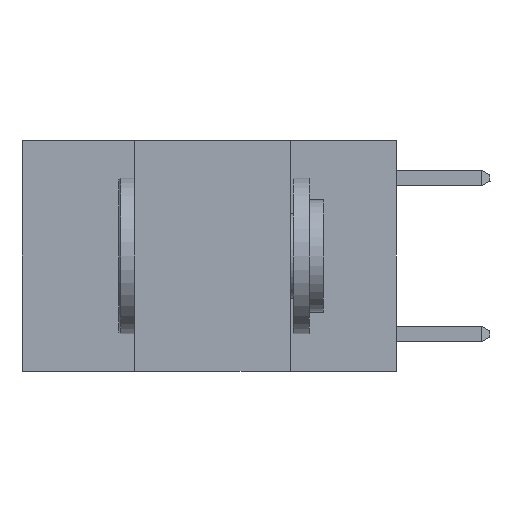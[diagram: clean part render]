
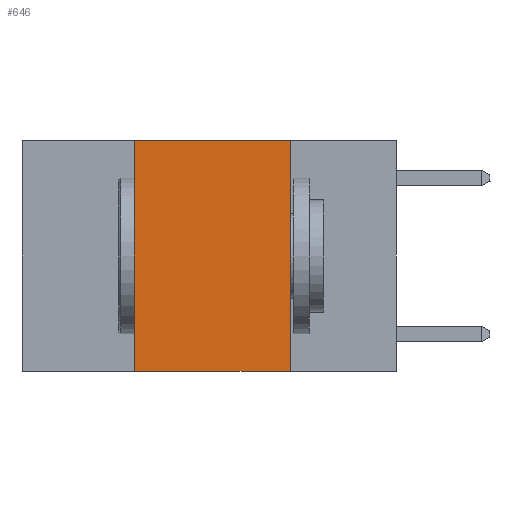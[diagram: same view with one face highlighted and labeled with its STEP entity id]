
A CAD part, left-side view. The second image highlights one B-rep face of the part: STEP entity #646.
In plain terms, the highlighted planar face has unit normal (-1, 0, 0).
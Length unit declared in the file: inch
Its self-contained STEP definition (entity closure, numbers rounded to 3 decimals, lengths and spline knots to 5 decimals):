
#167 = ORIENTED_EDGE ( 'NONE', *, *, #4504, .F. ) ;
#646 = ADVANCED_FACE ( 'NONE', ( #1214 ), #1374, .F. ) ;
#1214 = FACE_OUTER_BOUND ( 'NONE', #1961, .T. ) ;
#1374 = PLANE ( 'NONE',  #2691 ) ;
#1961 = EDGE_LOOP ( 'NONE', ( #9115, #9384, #167, #2032 ) ) ;
#2032 = ORIENTED_EDGE ( 'NONE', *, *, #2106, .T. ) ;
#2106 = EDGE_CURVE ( 'NONE', #10160, #10422, #9159, .T. ) ;
#2201 = VECTOR ( 'NONE', #3782, 39.37008 ) ;
#2255 = LINE ( 'NONE', #3208, #2201 ) ;
#2525 = EDGE_CURVE ( 'NONE', #10385, #5576, #7835, .T. ) ;
#2691 = AXIS2_PLACEMENT_3D ( 'NONE', #2803, #3462, #3307 ) ;
#2792 = CARTESIAN_POINT ( 'NONE',  ( 0., 0.42, 0. ) ) ;
#2803 = CARTESIAN_POINT ( 'NONE',  ( 0., 0.6, 0. ) ) ;
#3208 = CARTESIAN_POINT ( 'NONE',  ( 0., 0.42, 0. ) ) ;
#3307 = DIRECTION ( 'NONE',  ( 0., 0., -1. ) ) ;
#3462 = DIRECTION ( 'NONE',  ( 1., 0., 0. ) ) ;
#3782 = DIRECTION ( 'NONE',  ( 0., 0., 1. ) ) ;
#3823 = EDGE_CURVE ( 'NONE', #5576, #10422, #4259, .T. ) ;
#4041 = DIRECTION ( 'NONE',  ( 0., -1., 0. ) ) ;
#4053 = CARTESIAN_POINT ( 'NONE',  ( 0., 0.6, 0. ) ) ;
#4225 = VECTOR ( 'NONE', #5171, 39.37008 ) ;
#4259 = LINE ( 'NONE', #5472, #4225 ) ;
#4504 = EDGE_CURVE ( 'NONE', #10160, #10385, #2255, .T. ) ;
#5171 = DIRECTION ( 'NONE',  ( 0., 0., -1. ) ) ;
#5472 = CARTESIAN_POINT ( 'NONE',  ( 0., 0.17, 0. ) ) ;
#5576 = VERTEX_POINT ( 'NONE', #9936 ) ;
#6854 = CARTESIAN_POINT ( 'NONE',  ( 0., 0.17, -0.37 ) ) ;
#7814 = VECTOR ( 'NONE', #4041, 39.37008 ) ;
#7835 = LINE ( 'NONE', #4053, #7814 ) ;
#8167 = CARTESIAN_POINT ( 'NONE',  ( 0., 0.42, -0.37 ) ) ;
#8745 = DIRECTION ( 'NONE',  ( 0., -1., 0. ) ) ;
#8974 = CARTESIAN_POINT ( 'NONE',  ( 0., 0.6, -0.37 ) ) ;
#9115 = ORIENTED_EDGE ( 'NONE', *, *, #3823, .F. ) ;
#9121 = VECTOR ( 'NONE', #8745, 39.37008 ) ;
#9159 = LINE ( 'NONE', #8974, #9121 ) ;
#9384 = ORIENTED_EDGE ( 'NONE', *, *, #2525, .F. ) ;
#9936 = CARTESIAN_POINT ( 'NONE',  ( 0., 0.17, 0. ) ) ;
#10160 = VERTEX_POINT ( 'NONE', #8167 ) ;
#10385 = VERTEX_POINT ( 'NONE', #2792 ) ;
#10422 = VERTEX_POINT ( 'NONE', #6854 ) ;
